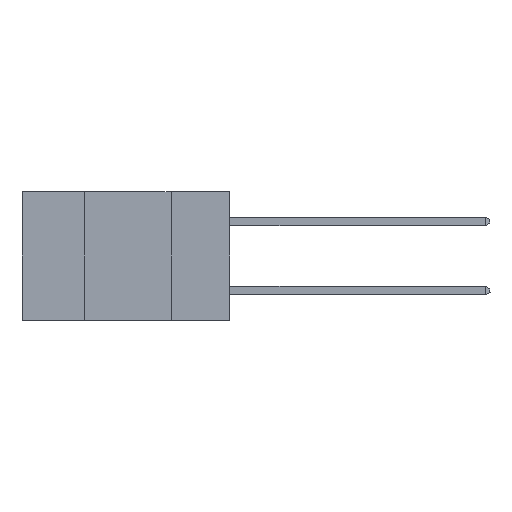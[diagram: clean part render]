
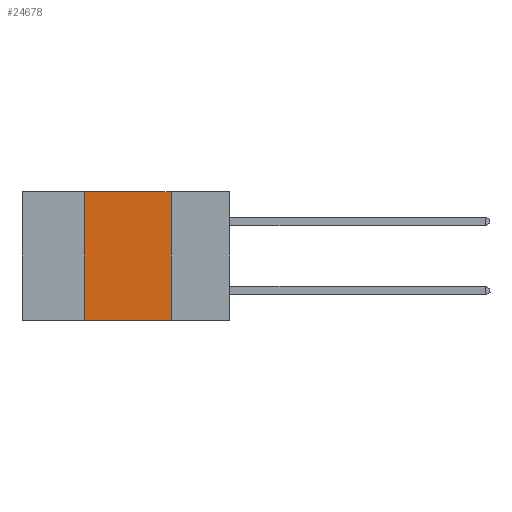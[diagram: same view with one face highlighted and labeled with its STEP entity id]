
A CAD part, left-side view. The second image highlights one B-rep face of the part: STEP entity #24678.
In plain terms, the highlighted planar face has unit normal (-1, 0, 0).
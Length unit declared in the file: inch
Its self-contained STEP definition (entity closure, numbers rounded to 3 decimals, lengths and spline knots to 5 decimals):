
#1140 = EDGE_CURVE ( 'NONE', #15702, #14003, #13038, .T. ) ;
#1447 = CARTESIAN_POINT ( 'NONE',  ( 0., 0.17, 0. ) ) ;
#1683 = DIRECTION ( 'NONE',  ( 0., 0., -1. ) ) ;
#1805 = DIRECTION ( 'NONE',  ( 0., 0., 1. ) ) ;
#2752 = AXIS2_PLACEMENT_3D ( 'NONE', #15462, #12951, #1683 ) ;
#2814 = CARTESIAN_POINT ( 'NONE',  ( 0., 0.42, 0. ) ) ;
#3857 = DIRECTION ( 'NONE',  ( 0., -1., 0. ) ) ;
#4915 = VERTEX_POINT ( 'NONE', #2814 ) ;
#6281 = ORIENTED_EDGE ( 'NONE', *, *, #20356, .T. ) ;
#6695 = ORIENTED_EDGE ( 'NONE', *, *, #1140, .F. ) ;
#7233 = VECTOR ( 'NONE', #8873, 39.37008 ) ;
#8873 = DIRECTION ( 'NONE',  ( 0., -1., 0. ) ) ;
#8983 = CARTESIAN_POINT ( 'NONE',  ( 0., 0.6, 0. ) ) ;
#11180 = CARTESIAN_POINT ( 'NONE',  ( 0., 0.17, -0.37 ) ) ;
#11774 = EDGE_LOOP ( 'NONE', ( #6695, #16626, #27532, #6281 ) ) ;
#12951 = DIRECTION ( 'NONE',  ( 1., 0., 0. ) ) ;
#13038 = LINE ( 'NONE', #1447, #24568 ) ;
#13992 = LINE ( 'NONE', #26662, #28405 ) ;
#14003 = VERTEX_POINT ( 'NONE', #11180 ) ;
#15048 = PLANE ( 'NONE',  #2752 ) ;
#15462 = CARTESIAN_POINT ( 'NONE',  ( 0., 0.6, 0. ) ) ;
#15702 = VERTEX_POINT ( 'NONE', #29452 ) ;
#15997 = LINE ( 'NONE', #24179, #16342 ) ;
#16342 = VECTOR ( 'NONE', #3857, 39.37008 ) ;
#16626 = ORIENTED_EDGE ( 'NONE', *, *, #22000, .F. ) ;
#20356 = EDGE_CURVE ( 'NONE', #24767, #14003, #15997, .T. ) ;
#22000 = EDGE_CURVE ( 'NONE', #4915, #15702, #29614, .T. ) ;
#24179 = CARTESIAN_POINT ( 'NONE',  ( 0., 0.6, -0.37 ) ) ;
#24568 = VECTOR ( 'NONE', #28937, 39.37008 ) ;
#24678 = ADVANCED_FACE ( 'NONE', ( #29475 ), #15048, .F. ) ;
#24767 = VERTEX_POINT ( 'NONE', #27269 ) ;
#26662 = CARTESIAN_POINT ( 'NONE',  ( 0., 0.42, 0. ) ) ;
#27269 = CARTESIAN_POINT ( 'NONE',  ( 0., 0.42, -0.37 ) ) ;
#27532 = ORIENTED_EDGE ( 'NONE', *, *, #28242, .F. ) ;
#28242 = EDGE_CURVE ( 'NONE', #24767, #4915, #13992, .T. ) ;
#28405 = VECTOR ( 'NONE', #1805, 39.37008 ) ;
#28937 = DIRECTION ( 'NONE',  ( 0., 0., -1. ) ) ;
#29452 = CARTESIAN_POINT ( 'NONE',  ( 0., 0.17, 0. ) ) ;
#29475 = FACE_OUTER_BOUND ( 'NONE', #11774, .T. ) ;
#29614 = LINE ( 'NONE', #8983, #7233 ) ;
